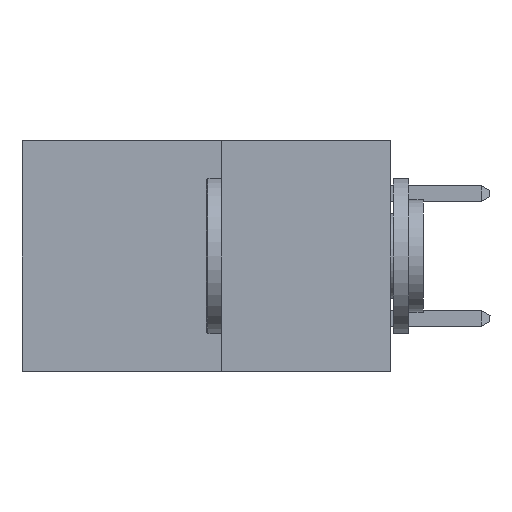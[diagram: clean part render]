
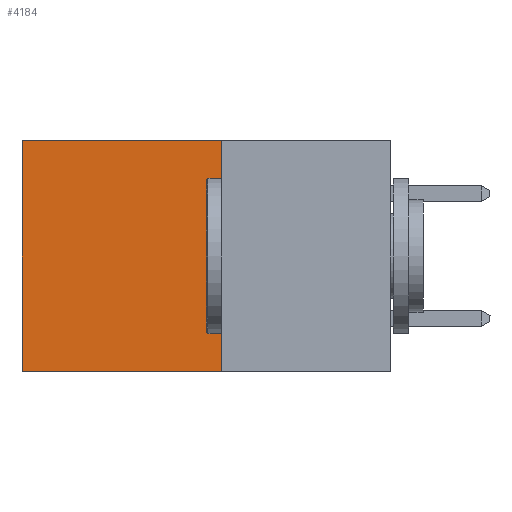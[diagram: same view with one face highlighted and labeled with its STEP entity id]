
A CAD part, left-side view. The second image highlights one B-rep face of the part: STEP entity #4184.
In plain terms, the highlighted planar face has unit normal (-1, 0, 0).
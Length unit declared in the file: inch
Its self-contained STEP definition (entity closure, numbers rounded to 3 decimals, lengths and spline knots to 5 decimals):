
#932 = VECTOR ( 'NONE', #5406, 39.37008 ) ;
#2341 = VECTOR ( 'NONE', #18980, 39.37008 ) ;
#2856 = CARTESIAN_POINT ( 'NONE',  ( 0.277, 0.59, -0.37 ) ) ;
#3764 = DIRECTION ( 'NONE',  ( 0., 0., -1. ) ) ;
#3770 = DIRECTION ( 'NONE',  ( 1., 0., 0. ) ) ;
#4014 = PLANE ( 'NONE',  #9379 ) ;
#4184 = ADVANCED_FACE ( 'NONE', ( #15231 ), #4014, .F. ) ;
#4741 = CARTESIAN_POINT ( 'NONE',  ( 0.277, 0.27, -0.37 ) ) ;
#4895 = EDGE_CURVE ( 'NONE', #7867, #20194, #19804, .T. ) ;
#5263 = CARTESIAN_POINT ( 'NONE',  ( 0.277, 0.27, -0.37 ) ) ;
#5406 = DIRECTION ( 'NONE',  ( 0., 1., 0. ) ) ;
#6335 = LINE ( 'NONE', #25297, #31609 ) ;
#6551 = EDGE_CURVE ( 'NONE', #13172, #7867, #20244, .T. ) ;
#7089 = VECTOR ( 'NONE', #10502, 39.37008 ) ;
#7867 = VERTEX_POINT ( 'NONE', #9566 ) ;
#9379 = AXIS2_PLACEMENT_3D ( 'NONE', #4741, #3770, #3764 ) ;
#9566 = CARTESIAN_POINT ( 'NONE',  ( 0.277, 0.27, -0.37 ) ) ;
#9839 = CARTESIAN_POINT ( 'NONE',  ( 0.277, 0.27, 0. ) ) ;
#10502 = DIRECTION ( 'NONE',  ( 0., 0., -1. ) ) ;
#10711 = CARTESIAN_POINT ( 'NONE',  ( 0.277, 0.27, -0.37 ) ) ;
#11035 = EDGE_CURVE ( 'NONE', #13172, #14573, #6335, .T. ) ;
#11094 = ORIENTED_EDGE ( 'NONE', *, *, #13671, .T. ) ;
#13172 = VERTEX_POINT ( 'NONE', #9839 ) ;
#13671 = EDGE_CURVE ( 'NONE', #14573, #20194, #22001, .T. ) ;
#13990 = ORIENTED_EDGE ( 'NONE', *, *, #11035, .T. ) ;
#14573 = VERTEX_POINT ( 'NONE', #16761 ) ;
#15231 = FACE_OUTER_BOUND ( 'NONE', #22973, .T. ) ;
#15977 = ORIENTED_EDGE ( 'NONE', *, *, #6551, .F. ) ;
#16517 = CARTESIAN_POINT ( 'NONE',  ( 0.277, 0.59, -0.37 ) ) ;
#16761 = CARTESIAN_POINT ( 'NONE',  ( 0.277, 0.59, 0. ) ) ;
#18980 = DIRECTION ( 'NONE',  ( 0., 0., -1. ) ) ;
#19804 = LINE ( 'NONE', #5263, #932 ) ;
#20194 = VERTEX_POINT ( 'NONE', #2856 ) ;
#20244 = LINE ( 'NONE', #10711, #7089 ) ;
#22001 = LINE ( 'NONE', #16517, #2341 ) ;
#22973 = EDGE_LOOP ( 'NONE', ( #11094, #29648, #15977, #13990 ) ) ;
#25297 = CARTESIAN_POINT ( 'NONE',  ( 0.277, 0.27, 0. ) ) ;
#25394 = DIRECTION ( 'NONE',  ( 0., 1., 0. ) ) ;
#29648 = ORIENTED_EDGE ( 'NONE', *, *, #4895, .F. ) ;
#31609 = VECTOR ( 'NONE', #25394, 39.37008 ) ;
